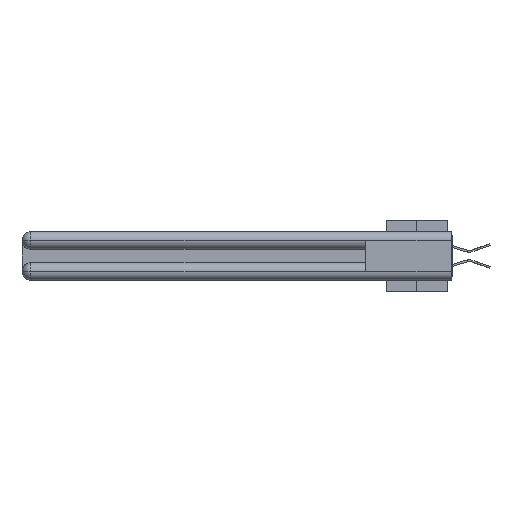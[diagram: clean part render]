
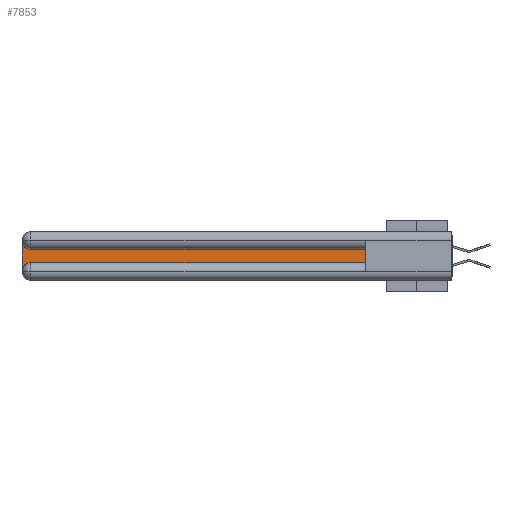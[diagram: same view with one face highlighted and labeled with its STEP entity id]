
A CAD part, left-side view. The second image highlights one B-rep face of the part: STEP entity #7853.
In plain terms, the highlighted planar face has unit normal (-1, 0, 0).
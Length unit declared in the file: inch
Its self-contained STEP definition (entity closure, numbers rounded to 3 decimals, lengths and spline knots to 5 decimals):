
#279 = CIRCLE ( 'NONE', #29282, 0.06 ) ;
#3355 = ORIENTED_EDGE ( 'NONE', *, *, #14747, .T. ) ;
#4746 = VERTEX_POINT ( 'NONE', #19957 ) ;
#5345 = DIRECTION ( 'NONE',  ( 1., 0., 0. ) ) ;
#5582 = DIRECTION ( 'NONE',  ( 1., 0., 0. ) ) ;
#6162 = DIRECTION ( 'NONE',  ( 0., 0., -1. ) ) ;
#7853 = ADVANCED_FACE ( 'NONE', ( #26865 ), #9537, .F. ) ;
#8159 = LINE ( 'NONE', #20445, #11289 ) ;
#8455 = VECTOR ( 'NONE', #41092, 39.37008 ) ;
#9227 = CARTESIAN_POINT ( 'NONE',  ( 0.075, 2.94, -0.0625 ) ) ;
#9537 = PLANE ( 'NONE',  #34427 ) ;
#10159 = ORIENTED_EDGE ( 'NONE', *, *, #33445, .T. ) ;
#11284 = ORIENTED_EDGE ( 'NONE', *, *, #36306, .T. ) ;
#11289 = VECTOR ( 'NONE', #27261, 39.37008 ) ;
#12147 = DIRECTION ( 'NONE',  ( 0., 0., -1. ) ) ;
#12162 = VERTEX_POINT ( 'NONE', #42008 ) ;
#13904 = ORIENTED_EDGE ( 'NONE', *, *, #27883, .T. ) ;
#14420 = CARTESIAN_POINT ( 'NONE',  ( 0.075, 3., -0.0625 ) ) ;
#14747 = EDGE_CURVE ( 'NONE', #4746, #12162, #8159, .T. ) ;
#14840 = VERTEX_POINT ( 'NONE', #21460 ) ;
#15542 = VERTEX_POINT ( 'NONE', #27649 ) ;
#16198 = LINE ( 'NONE', #24326, #8455 ) ;
#16309 = VECTOR ( 'NONE', #12147, 39.37008 ) ;
#19183 = CARTESIAN_POINT ( 'NONE',  ( 0.075, 3., -0.2775 ) ) ;
#19957 = CARTESIAN_POINT ( 'NONE',  ( 0.075, 0.6, -0.2175 ) ) ;
#20156 = DIRECTION ( 'NONE',  ( 0., 1., 0. ) ) ;
#20445 = CARTESIAN_POINT ( 'NONE',  ( 0.075, 0.6, -0.2175 ) ) ;
#21460 = CARTESIAN_POINT ( 'NONE',  ( 0.075, 2.94, -0.1225 ) ) ;
#23095 = CARTESIAN_POINT ( 'NONE',  ( 0.075, 3., -0.1225 ) ) ;
#23824 = DIRECTION ( 'NONE',  ( 1., 0., 0. ) ) ;
#23934 = CARTESIAN_POINT ( 'NONE',  ( 0.075, 0.6, -0.1225 ) ) ;
#24326 = CARTESIAN_POINT ( 'NONE',  ( 0.075, 0.6, -0.2175 ) ) ;
#25460 = EDGE_CURVE ( 'NONE', #35783, #15542, #279, .T. ) ;
#26865 = FACE_OUTER_BOUND ( 'NONE', #32258, .T. ) ;
#27030 = VECTOR ( 'NONE', #20156, 39.37008 ) ;
#27261 = DIRECTION ( 'NONE',  ( 0., 0., 1. ) ) ;
#27649 = CARTESIAN_POINT ( 'NONE',  ( 0.075, 2.94, -0.2175 ) ) ;
#27883 = EDGE_CURVE ( 'NONE', #42156, #35783, #42861, .T. ) ;
#28500 = DIRECTION ( 'NONE',  ( 0., 0., -1. ) ) ;
#28517 = CARTESIAN_POINT ( 'NONE',  ( 0.075, 3., -0.2175 ) ) ;
#28745 = CARTESIAN_POINT ( 'NONE',  ( 0.075, 2.94, -0.2775 ) ) ;
#29282 = AXIS2_PLACEMENT_3D ( 'NONE', #28745, #5582, #31559 ) ;
#29914 = EDGE_CURVE ( 'NONE', #12162, #14840, #40597, .T. ) ;
#31559 = DIRECTION ( 'NONE',  ( 0., 0., -1. ) ) ;
#31988 = CIRCLE ( 'NONE', #34290, 0.06 ) ;
#32258 = EDGE_LOOP ( 'NONE', ( #40253, #11284, #13904, #40273, #10159, #3355 ) ) ;
#33445 = EDGE_CURVE ( 'NONE', #15542, #4746, #16198, .T. ) ;
#34290 = AXIS2_PLACEMENT_3D ( 'NONE', #9227, #5345, #28500 ) ;
#34427 = AXIS2_PLACEMENT_3D ( 'NONE', #23095, #23824, #6162 ) ;
#35783 = VERTEX_POINT ( 'NONE', #19183 ) ;
#36306 = EDGE_CURVE ( 'NONE', #14840, #42156, #31988, .T. ) ;
#40253 = ORIENTED_EDGE ( 'NONE', *, *, #29914, .T. ) ;
#40273 = ORIENTED_EDGE ( 'NONE', *, *, #25460, .T. ) ;
#40597 = LINE ( 'NONE', #23934, #27030 ) ;
#41092 = DIRECTION ( 'NONE',  ( 0., -1., 0. ) ) ;
#42008 = CARTESIAN_POINT ( 'NONE',  ( 0.075, 0.6, -0.1225 ) ) ;
#42156 = VERTEX_POINT ( 'NONE', #14420 ) ;
#42861 = LINE ( 'NONE', #28517, #16309 ) ;
